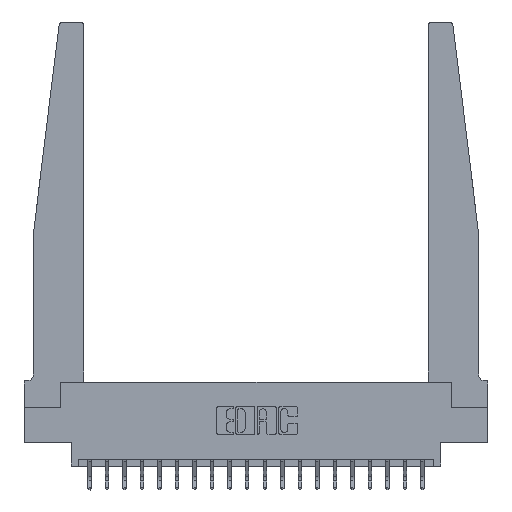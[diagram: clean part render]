
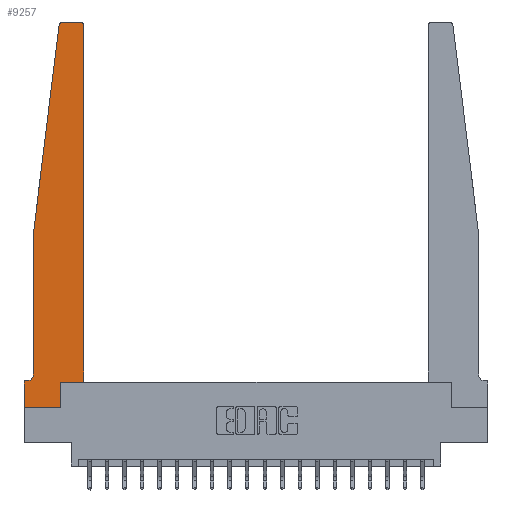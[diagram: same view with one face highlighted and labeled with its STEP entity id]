
A CAD part, top view. The second image highlights one B-rep face of the part: STEP entity #9257.
In plain terms, the highlighted planar face has unit normal (0, 0, 1).
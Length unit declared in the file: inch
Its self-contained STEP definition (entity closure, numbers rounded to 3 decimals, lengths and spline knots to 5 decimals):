
#31 = ORIENTED_EDGE ( 'NONE', *, *, #7737, .T. ) ;
#38 = FACE_OUTER_BOUND ( 'NONE', #19407, .T. ) ;
#160 = CARTESIAN_POINT ( 'NONE',  ( 0.425, 2.72, 0.37 ) ) ;
#492 = CARTESIAN_POINT ( 'NONE',  ( 0., 0., 0.37 ) ) ;
#535 = DIRECTION ( 'NONE',  ( 1., 0., 0. ) ) ;
#678 = CARTESIAN_POINT ( 'NONE',  ( 0.25, 2.75, 0.37 ) ) ;
#906 = CARTESIAN_POINT ( 'NONE',  ( 0., 0.1875, 0.37 ) ) ;
#1091 = CARTESIAN_POINT ( 'NONE',  ( 0.065, 1.25, 0.37 ) ) ;
#2197 = CARTESIAN_POINT ( 'NONE',  ( 0.015, 0.1875, 0.37 ) ) ;
#2241 = DIRECTION ( 'NONE',  ( 1., 0., 0. ) ) ;
#2245 = ORIENTED_EDGE ( 'NONE', *, *, #9974, .T. ) ;
#2313 = DIRECTION ( 'NONE',  ( -1., 0., 0. ) ) ;
#2563 = EDGE_CURVE ( 'NONE', #7806, #19500, #9310, .T. ) ;
#2892 = LINE ( 'NONE', #3077, #11145 ) ;
#2960 = ORIENTED_EDGE ( 'NONE', *, *, #15376, .T. ) ;
#3002 = DIRECTION ( 'NONE',  ( 1., 0., 0. ) ) ;
#3077 = CARTESIAN_POINT ( 'NONE',  ( 0.425, 0.18, 0.37 ) ) ;
#3446 = CIRCLE ( 'NONE', #9978, 0.05 ) ;
#3884 = VERTEX_POINT ( 'NONE', #10706 ) ;
#4148 = LINE ( 'NONE', #678, #16795 ) ;
#4276 = CARTESIAN_POINT ( 'NONE',  ( 0.065, 1.25, 0.37 ) ) ;
#4505 = DIRECTION ( 'NONE',  ( 0., 0., -1. ) ) ;
#4815 = CARTESIAN_POINT ( 'NONE',  ( 0., 0., 0.37 ) ) ;
#4826 = ORIENTED_EDGE ( 'NONE', *, *, #17470, .T. ) ;
#4889 = VECTOR ( 'NONE', #15994, 39.37008 ) ;
#5181 = CARTESIAN_POINT ( 'NONE',  ( 0.425, 0.18, 0.37 ) ) ;
#5597 = CIRCLE ( 'NONE', #14854, 0.03 ) ;
#6025 = DIRECTION ( 'NONE',  ( -1., 0., 0. ) ) ;
#6029 = VERTEX_POINT ( 'NONE', #14381 ) ;
#6075 = LINE ( 'NONE', #15921, #15357 ) ;
#6449 = DIRECTION ( 'NONE',  ( 0., 1., 0. ) ) ;
#6493 = DIRECTION ( 'NONE',  ( 1., 0., 0. ) ) ;
#6581 = ORIENTED_EDGE ( 'NONE', *, *, #7318, .T. ) ;
#6777 = ORIENTED_EDGE ( 'NONE', *, *, #7252, .T. ) ;
#7252 = EDGE_CURVE ( 'NONE', #19500, #12694, #8285, .T. ) ;
#7318 = EDGE_CURVE ( 'NONE', #12694, #8009, #2892, .T. ) ;
#7728 = VERTEX_POINT ( 'NONE', #4276 ) ;
#7737 = EDGE_CURVE ( 'NONE', #7728, #14165, #13719, .T. ) ;
#7792 = CARTESIAN_POINT ( 'NONE',  ( 0.27653, 2.72, 0.37 ) ) ;
#7806 = VERTEX_POINT ( 'NONE', #12733 ) ;
#7927 = EDGE_CURVE ( 'NONE', #15851, #7806, #14982, .T. ) ;
#8009 = VERTEX_POINT ( 'NONE', #160 ) ;
#8285 = LINE ( 'NONE', #16147, #20821 ) ;
#8709 = DIRECTION ( 'NONE',  ( 0., -1., 0. ) ) ;
#8744 = CARTESIAN_POINT ( 'NONE',  ( 0.065, 1.25, 0.37 ) ) ;
#8783 = CARTESIAN_POINT ( 'NONE',  ( 0.24675, 2.72367, 0.37 ) ) ;
#9031 = ORIENTED_EDGE ( 'NONE', *, *, #13390, .T. ) ;
#9257 = ADVANCED_FACE ( 'NONE', ( #38 ), #16989, .T. ) ;
#9310 = LINE ( 'NONE', #9345, #4889 ) ;
#9345 = CARTESIAN_POINT ( 'NONE',  ( 0.2605, 0.18, 0.37 ) ) ;
#9452 = DIRECTION ( 'NONE',  ( 1., 0., 0. ) ) ;
#9767 = ORIENTED_EDGE ( 'NONE', *, *, #20037, .T. ) ;
#9974 = EDGE_CURVE ( 'NONE', #3884, #13422, #5597, .T. ) ;
#9978 = AXIS2_PLACEMENT_3D ( 'NONE', #14406, #4505, #16067 ) ;
#10341 = DIRECTION ( 'NONE',  ( 0., 0., 1. ) ) ;
#10470 = VERTEX_POINT ( 'NONE', #906 ) ;
#10593 = CARTESIAN_POINT ( 'NONE',  ( 0.065, 0.2375, 0.37 ) ) ;
#10706 = CARTESIAN_POINT ( 'NONE',  ( 0.27653, 2.75, 0.37 ) ) ;
#10919 = DIRECTION ( 'NONE',  ( 0., -1., 0. ) ) ;
#11145 = VECTOR ( 'NONE', #6449, 39.37008 ) ;
#12095 = DIRECTION ( 'NONE',  ( 0., 0., 1. ) ) ;
#12694 = VERTEX_POINT ( 'NONE', #5181 ) ;
#12733 = CARTESIAN_POINT ( 'NONE',  ( 0.2605, 0., 0.37 ) ) ;
#13390 = EDGE_CURVE ( 'NONE', #10470, #15851, #18594, .T. ) ;
#13422 = VERTEX_POINT ( 'NONE', #8783 ) ;
#13491 = AXIS2_PLACEMENT_3D ( 'NONE', #15327, #12095, #2241 ) ;
#13661 = VECTOR ( 'NONE', #18593, 39.37008 ) ;
#13679 = ORIENTED_EDGE ( 'NONE', *, *, #2563, .T. ) ;
#13719 = LINE ( 'NONE', #1091, #17575 ) ;
#14038 = EDGE_CURVE ( 'NONE', #8009, #6029, #16039, .T. ) ;
#14165 = VERTEX_POINT ( 'NONE', #10593 ) ;
#14259 = VECTOR ( 'NONE', #8709, 39.37008 ) ;
#14381 = CARTESIAN_POINT ( 'NONE',  ( 0.395, 2.75, 0.37 ) ) ;
#14406 = CARTESIAN_POINT ( 'NONE',  ( 0.015, 0.2375, 0.37 ) ) ;
#14480 = VECTOR ( 'NONE', #6493, 39.37008 ) ;
#14728 = CARTESIAN_POINT ( 'NONE',  ( 0., 0., 0.37 ) ) ;
#14740 = CARTESIAN_POINT ( 'NONE',  ( 0.2605, 0.18, 0.37 ) ) ;
#14770 = ORIENTED_EDGE ( 'NONE', *, *, #7927, .T. ) ;
#14854 = AXIS2_PLACEMENT_3D ( 'NONE', #7792, #19274, #9452 ) ;
#14982 = LINE ( 'NONE', #14728, #14480 ) ;
#15327 = CARTESIAN_POINT ( 'NONE',  ( 0., 0.1875, 0.37 ) ) ;
#15357 = VECTOR ( 'NONE', #6025, 39.37008 ) ;
#15376 = EDGE_CURVE ( 'NONE', #13422, #7728, #17512, .T. ) ;
#15455 = AXIS2_PLACEMENT_3D ( 'NONE', #20128, #10341, #535 ) ;
#15851 = VERTEX_POINT ( 'NONE', #4815 ) ;
#15921 = CARTESIAN_POINT ( 'NONE',  ( 0.065, 0.1875, 0.37 ) ) ;
#15994 = DIRECTION ( 'NONE',  ( 0., 1., 0. ) ) ;
#16039 = CIRCLE ( 'NONE', #15455, 0.03 ) ;
#16067 = DIRECTION ( 'NONE',  ( -1., 0., 0. ) ) ;
#16104 = VERTEX_POINT ( 'NONE', #2197 ) ;
#16147 = CARTESIAN_POINT ( 'NONE',  ( 0.425, 0.18, 0.37 ) ) ;
#16795 = VECTOR ( 'NONE', #2313, 39.37008 ) ;
#16989 = PLANE ( 'NONE',  #13491 ) ;
#17470 = EDGE_CURVE ( 'NONE', #16104, #10470, #6075, .T. ) ;
#17512 = LINE ( 'NONE', #8744, #13661 ) ;
#17575 = VECTOR ( 'NONE', #10919, 39.37008 ) ;
#18456 = ORIENTED_EDGE ( 'NONE', *, *, #19339, .T. ) ;
#18593 = DIRECTION ( 'NONE',  ( -0.122, -0.992, 0. ) ) ;
#18594 = LINE ( 'NONE', #492, #14259 ) ;
#19274 = DIRECTION ( 'NONE',  ( 0., 0., 1. ) ) ;
#19339 = EDGE_CURVE ( 'NONE', #14165, #16104, #3446, .T. ) ;
#19364 = ORIENTED_EDGE ( 'NONE', *, *, #14038, .T. ) ;
#19407 = EDGE_LOOP ( 'NONE', ( #9767, #2245, #2960, #31, #18456, #4826, #9031, #14770, #13679, #6777, #6581, #19364 ) ) ;
#19500 = VERTEX_POINT ( 'NONE', #14740 ) ;
#20037 = EDGE_CURVE ( 'NONE', #6029, #3884, #4148, .T. ) ;
#20128 = CARTESIAN_POINT ( 'NONE',  ( 0.395, 2.72, 0.37 ) ) ;
#20821 = VECTOR ( 'NONE', #3002, 39.37008 ) ;
